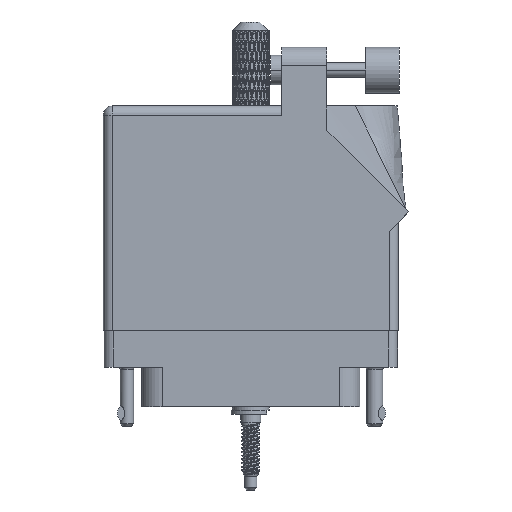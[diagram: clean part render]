
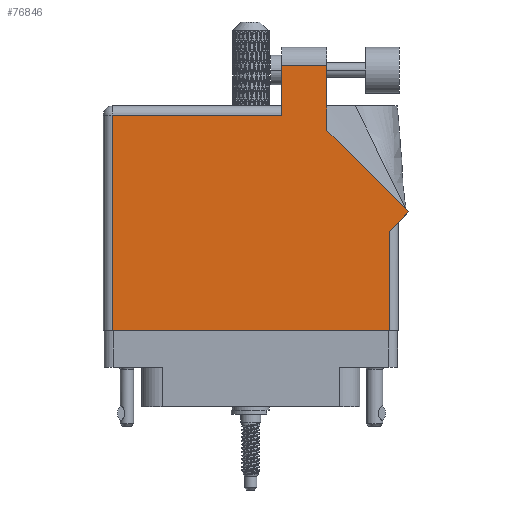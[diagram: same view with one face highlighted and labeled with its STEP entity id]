
A CAD part, front view. The second image highlights one B-rep face of the part: STEP entity #76846.
In plain terms, the highlighted face is planar.
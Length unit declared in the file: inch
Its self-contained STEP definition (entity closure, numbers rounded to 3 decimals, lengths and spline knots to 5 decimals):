
#5080 = VERTEX_POINT ( 'NONE', #68101 ) ;
#5373 = VECTOR ( 'NONE', #100734, 39.37008 ) ;
#7086 = EDGE_CURVE ( 'NONE', #14437, #5080, #63017, .T. ) ;
#8639 = DIRECTION ( 'NONE',  ( -0.707, 0.707, 0. ) ) ;
#12049 = VECTOR ( 'NONE', #95180, 39.37008 ) ;
#13809 = ORIENTED_EDGE ( 'NONE', *, *, #53290, .T. ) ;
#14437 = VERTEX_POINT ( 'NONE', #94090 ) ;
#15948 = VERTEX_POINT ( 'NONE', #81375 ) ;
#20408 = EDGE_CURVE ( 'NONE', #38739, #15948, #79146, .T. ) ;
#20982 = CARTESIAN_POINT ( 'NONE',  ( -1.005, 1.43, 0.455 ) ) ;
#21205 = VERTEX_POINT ( 'NONE', #90300 ) ;
#21866 = ORIENTED_EDGE ( 'NONE', *, *, #82410, .T. ) ;
#23235 = ORIENTED_EDGE ( 'NONE', *, *, #7086, .T. ) ;
#24888 = CARTESIAN_POINT ( 'NONE',  ( 0.519, 1.705, 0.455 ) ) ;
#24986 = CARTESIAN_POINT ( 'NONE',  ( 1.07571, 0.70771, 0.455 ) ) ;
#27783 = ORIENTED_EDGE ( 'NONE', *, *, #20408, .T. ) ;
#27834 = VECTOR ( 'NONE', #79285, 39.37008 ) ;
#29086 = DIRECTION ( 'NONE',  ( 0., -1., 0. ) ) ;
#29760 = CARTESIAN_POINT ( 'NONE',  ( -0.943, 1.368, 0.455 ) ) ;
#31845 = VECTOR ( 'NONE', #81212, 39.37008 ) ;
#32642 = CARTESIAN_POINT ( 'NONE',  ( -1.005, 1.368, 0.455 ) ) ;
#33477 = ORIENTED_EDGE ( 'NONE', *, *, #113684, .T. ) ;
#34278 = CARTESIAN_POINT ( 'NONE',  ( 1.07571, 0.70771, 0.455 ) ) ;
#36393 = VECTOR ( 'NONE', #96579, 39.37008 ) ;
#37348 = ORIENTED_EDGE ( 'NONE', *, *, #49028, .T. ) ;
#38397 = DIRECTION ( 'NONE',  ( 0., 0., -1. ) ) ;
#38739 = VERTEX_POINT ( 'NONE', #24888 ) ;
#39201 = LINE ( 'NONE', #78694, #36393 ) ;
#41204 = VECTOR ( 'NONE', #29086, 39.37008 ) ;
#46507 = EDGE_CURVE ( 'NONE', #107171, #38739, #97163, .T. ) ;
#46756 = ORIENTED_EDGE ( 'NONE', *, *, #99647, .T. ) ;
#47048 = CARTESIAN_POINT ( 'NONE',  ( -1.005, -0.1, 0.455 ) ) ;
#47605 = CARTESIAN_POINT ( 'NONE',  ( 0.212, 1.43, 0.455 ) ) ;
#49028 = EDGE_CURVE ( 'NONE', #15948, #109180, #110583, .T. ) ;
#49388 = ORIENTED_EDGE ( 'NONE', *, *, #83226, .T. ) ;
#53192 = VERTEX_POINT ( 'NONE', #24986 ) ;
#53290 = EDGE_CURVE ( 'NONE', #53192, #107171, #103228, .T. ) ;
#54588 = AXIS2_PLACEMENT_3D ( 'NONE', #20982, #38397, #100573 ) ;
#57789 = CARTESIAN_POINT ( 'NONE',  ( 1.005, 0.637, 0.455 ) ) ;
#62546 = CARTESIAN_POINT ( 'NONE',  ( 0.212, 1.705, 0.455 ) ) ;
#63017 = LINE ( 'NONE', #67090, #101976 ) ;
#63270 = CARTESIAN_POINT ( 'NONE',  ( 0.212, 1.368, 0.455 ) ) ;
#65437 = EDGE_LOOP ( 'NONE', ( #107517, #27783, #37348, #49388, #33477, #46756, #23235, #21866, #13809 ) ) ;
#66261 = LINE ( 'NONE', #57789, #83018 ) ;
#66681 = DIRECTION ( 'NONE',  ( 0.707, 0.707, 0. ) ) ;
#67090 = CARTESIAN_POINT ( 'NONE',  ( 0.943, 0.637, 0.455 ) ) ;
#67987 = LINE ( 'NONE', #47048, #5373 ) ;
#68101 = CARTESIAN_POINT ( 'NONE',  ( 0.943, 0.575, 0.455 ) ) ;
#73943 = FACE_OUTER_BOUND ( 'NONE', #65437, .T. ) ;
#76846 = ADVANCED_FACE ( 'NONE', ( #73943 ), #91630, .F. ) ;
#78694 = CARTESIAN_POINT ( 'NONE',  ( -0.943, -0.1, 0.455 ) ) ;
#79146 = LINE ( 'NONE', #62546, #27834 ) ;
#79285 = DIRECTION ( 'NONE',  ( -1., 0., 0. ) ) ;
#80140 = LINE ( 'NONE', #32642, #12049 ) ;
#81212 = DIRECTION ( 'NONE',  ( 0., 1., 0. ) ) ;
#81375 = CARTESIAN_POINT ( 'NONE',  ( 0.212, 1.705, 0.455 ) ) ;
#82410 = EDGE_CURVE ( 'NONE', #5080, #53192, #66261, .T. ) ;
#83018 = VECTOR ( 'NONE', #66681, 39.37008 ) ;
#83226 = EDGE_CURVE ( 'NONE', #109180, #114553, #80140, .T. ) ;
#84716 = CARTESIAN_POINT ( 'NONE',  ( 0.519, 1.26442, 0.455 ) ) ;
#90159 = CARTESIAN_POINT ( 'NONE',  ( 0.519, 1.26442, 0.455 ) ) ;
#90300 = CARTESIAN_POINT ( 'NONE',  ( -0.943, -0.1, 0.455 ) ) ;
#91630 = PLANE ( 'NONE',  #54588 ) ;
#94090 = CARTESIAN_POINT ( 'NONE',  ( 0.943, -0.1, 0.455 ) ) ;
#95180 = DIRECTION ( 'NONE',  ( -1., 0., 0. ) ) ;
#96275 = VECTOR ( 'NONE', #8639, 39.37008 ) ;
#96579 = DIRECTION ( 'NONE',  ( 0., -1., 0. ) ) ;
#97163 = LINE ( 'NONE', #90159, #31845 ) ;
#99647 = EDGE_CURVE ( 'NONE', #21205, #14437, #67987, .T. ) ;
#100573 = DIRECTION ( 'NONE',  ( -1., 0., 0. ) ) ;
#100734 = DIRECTION ( 'NONE',  ( 1., 0., 0. ) ) ;
#101976 = VECTOR ( 'NONE', #104856, 39.37008 ) ;
#103228 = LINE ( 'NONE', #34278, #96275 ) ;
#104856 = DIRECTION ( 'NONE',  ( 0., 1., 0. ) ) ;
#107171 = VERTEX_POINT ( 'NONE', #84716 ) ;
#107517 = ORIENTED_EDGE ( 'NONE', *, *, #46507, .T. ) ;
#109180 = VERTEX_POINT ( 'NONE', #63270 ) ;
#110583 = LINE ( 'NONE', #47605, #41204 ) ;
#113684 = EDGE_CURVE ( 'NONE', #114553, #21205, #39201, .T. ) ;
#114553 = VERTEX_POINT ( 'NONE', #29760 ) ;
